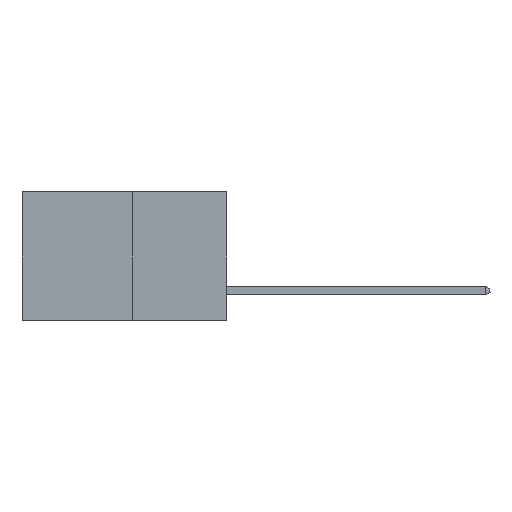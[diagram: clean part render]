
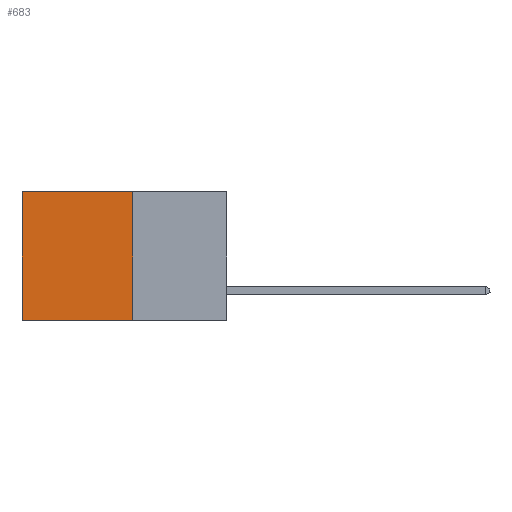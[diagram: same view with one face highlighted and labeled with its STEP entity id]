
A CAD part, left-side view. The second image highlights one B-rep face of the part: STEP entity #683.
In plain terms, the highlighted planar face has unit normal (-1, 0, 0).
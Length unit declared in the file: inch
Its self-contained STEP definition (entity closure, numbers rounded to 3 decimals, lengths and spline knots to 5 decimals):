
#178 = CARTESIAN_POINT ( 'NONE',  ( 0.277, 0.27, -0.37 ) ) ;
#416 = ORIENTED_EDGE ( 'NONE', *, *, #2776, .T. ) ;
#425 = DIRECTION ( 'NONE',  ( 0., 0., -1. ) ) ;
#683 = ADVANCED_FACE ( 'NONE', ( #5066 ), #1806, .F. ) ;
#1320 = CARTESIAN_POINT ( 'NONE',  ( 0.277, 0.27, -0.37 ) ) ;
#1806 = PLANE ( 'NONE',  #6722 ) ;
#1991 = EDGE_CURVE ( 'NONE', #2813, #7838, #5723, .T. ) ;
#2276 = CARTESIAN_POINT ( 'NONE',  ( 0.277, 0.59, -0.37 ) ) ;
#2343 = EDGE_CURVE ( 'NONE', #7838, #5087, #2395, .T. ) ;
#2395 = LINE ( 'NONE', #178, #6008 ) ;
#2466 = ORIENTED_EDGE ( 'NONE', *, *, #3341, .T. ) ;
#2730 = CARTESIAN_POINT ( 'NONE',  ( 0.277, 0.27, -0.37 ) ) ;
#2776 = EDGE_CURVE ( 'NONE', #2813, #5223, #5389, .T. ) ;
#2813 = VERTEX_POINT ( 'NONE', #7712 ) ;
#3337 = LINE ( 'NONE', #8533, #5068 ) ;
#3341 = EDGE_CURVE ( 'NONE', #5223, #5087, #3337, .T. ) ;
#3476 = VECTOR ( 'NONE', #7459, 39.37008 ) ;
#4051 = EDGE_LOOP ( 'NONE', ( #2466, #6266, #7897, #416 ) ) ;
#4549 = DIRECTION ( 'NONE',  ( 0., 0., -1. ) ) ;
#5066 = FACE_OUTER_BOUND ( 'NONE', #4051, .T. ) ;
#5068 = VECTOR ( 'NONE', #425, 39.37008 ) ;
#5087 = VERTEX_POINT ( 'NONE', #2276 ) ;
#5223 = VERTEX_POINT ( 'NONE', #8471 ) ;
#5389 = LINE ( 'NONE', #8040, #3476 ) ;
#5723 = LINE ( 'NONE', #1320, #8797 ) ;
#6008 = VECTOR ( 'NONE', #7932, 39.37008 ) ;
#6014 = DIRECTION ( 'NONE',  ( 0., 0., -1. ) ) ;
#6266 = ORIENTED_EDGE ( 'NONE', *, *, #2343, .F. ) ;
#6722 = AXIS2_PLACEMENT_3D ( 'NONE', #7939, #6754, #4549 ) ;
#6754 = DIRECTION ( 'NONE',  ( 1., 0., 0. ) ) ;
#7459 = DIRECTION ( 'NONE',  ( 0., 1., 0. ) ) ;
#7712 = CARTESIAN_POINT ( 'NONE',  ( 0.277, 0.27, 0. ) ) ;
#7838 = VERTEX_POINT ( 'NONE', #2730 ) ;
#7897 = ORIENTED_EDGE ( 'NONE', *, *, #1991, .F. ) ;
#7932 = DIRECTION ( 'NONE',  ( 0., 1., 0. ) ) ;
#7939 = CARTESIAN_POINT ( 'NONE',  ( 0.277, 0.27, -0.37 ) ) ;
#8040 = CARTESIAN_POINT ( 'NONE',  ( 0.277, 0.27, 0. ) ) ;
#8471 = CARTESIAN_POINT ( 'NONE',  ( 0.277, 0.59, 0. ) ) ;
#8533 = CARTESIAN_POINT ( 'NONE',  ( 0.277, 0.59, -0.37 ) ) ;
#8797 = VECTOR ( 'NONE', #6014, 39.37008 ) ;
